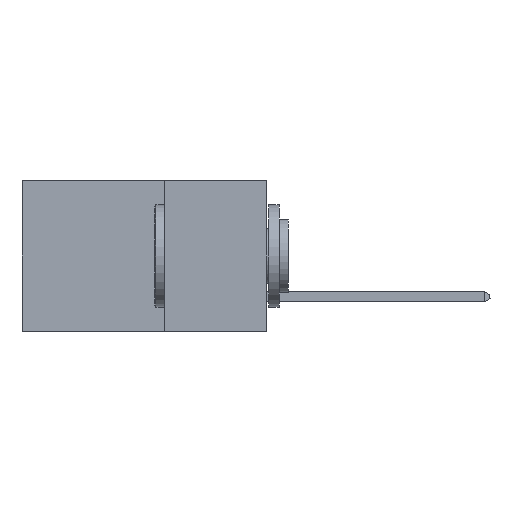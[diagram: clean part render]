
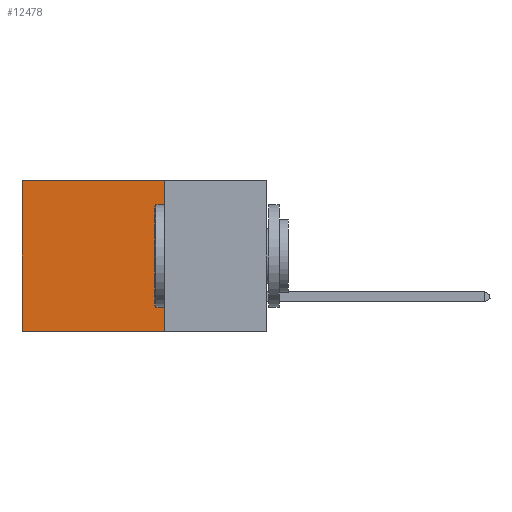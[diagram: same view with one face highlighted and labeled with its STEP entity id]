
A CAD part, left-side view. The second image highlights one B-rep face of the part: STEP entity #12478.
In plain terms, the highlighted planar face has unit normal (-1, 0, 0).
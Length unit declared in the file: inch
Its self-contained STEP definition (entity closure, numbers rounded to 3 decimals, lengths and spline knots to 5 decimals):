
#272 = DIRECTION ( 'NONE',  ( 0., 0., -1. ) ) ;
#1914 = PLANE ( 'NONE',  #24032 ) ;
#2000 = ORIENTED_EDGE ( 'NONE', *, *, #19717, .F. ) ;
#2892 = ORIENTED_EDGE ( 'NONE', *, *, #3190, .T. ) ;
#2979 = EDGE_CURVE ( 'NONE', #3474, #3676, #6004, .T. ) ;
#3190 = EDGE_CURVE ( 'NONE', #6959, #7015, #4786, .T. ) ;
#3474 = VERTEX_POINT ( 'NONE', #22950 ) ;
#3676 = VERTEX_POINT ( 'NONE', #20092 ) ;
#4786 = LINE ( 'NONE', #16646, #17984 ) ;
#4803 = VECTOR ( 'NONE', #5857, 39.37008 ) ;
#5398 = VECTOR ( 'NONE', #21744, 39.37008 ) ;
#5857 = DIRECTION ( 'NONE',  ( 0., 1., 0. ) ) ;
#5911 = CARTESIAN_POINT ( 'NONE',  ( 0.2875, 0.25, 0. ) ) ;
#6004 = LINE ( 'NONE', #17794, #5398 ) ;
#6959 = VERTEX_POINT ( 'NONE', #11608 ) ;
#7015 = VERTEX_POINT ( 'NONE', #21011 ) ;
#10780 = EDGE_CURVE ( 'NONE', #3474, #6959, #21262, .T. ) ;
#11608 = CARTESIAN_POINT ( 'NONE',  ( 0.2875, 0.6, 0. ) ) ;
#12478 = ADVANCED_FACE ( 'NONE', ( #21173 ), #1914, .F. ) ;
#15724 = DIRECTION ( 'NONE',  ( 0., 1., 0. ) ) ;
#16546 = VECTOR ( 'NONE', #15724, 39.37008 ) ;
#16646 = CARTESIAN_POINT ( 'NONE',  ( 0.2875, 0.6, 0. ) ) ;
#17124 = LINE ( 'NONE', #21621, #16546 ) ;
#17246 = ORIENTED_EDGE ( 'NONE', *, *, #10780, .T. ) ;
#17794 = CARTESIAN_POINT ( 'NONE',  ( 0.2875, 0.25, 0. ) ) ;
#17984 = VECTOR ( 'NONE', #22319, 39.37008 ) ;
#18734 = CARTESIAN_POINT ( 'NONE',  ( 0.2875, 0.25, 0. ) ) ;
#19096 = EDGE_LOOP ( 'NONE', ( #2892, #2000, #21598, #17246 ) ) ;
#19717 = EDGE_CURVE ( 'NONE', #3676, #7015, #17124, .T. ) ;
#20092 = CARTESIAN_POINT ( 'NONE',  ( 0.2875, 0.25, -0.37 ) ) ;
#20772 = DIRECTION ( 'NONE',  ( 1., 0., 0. ) ) ;
#21011 = CARTESIAN_POINT ( 'NONE',  ( 0.2875, 0.6, -0.37 ) ) ;
#21173 = FACE_OUTER_BOUND ( 'NONE', #19096, .T. ) ;
#21262 = LINE ( 'NONE', #18734, #4803 ) ;
#21598 = ORIENTED_EDGE ( 'NONE', *, *, #2979, .F. ) ;
#21621 = CARTESIAN_POINT ( 'NONE',  ( 0.2875, 0.25, -0.37 ) ) ;
#21744 = DIRECTION ( 'NONE',  ( 0., 0., -1. ) ) ;
#22319 = DIRECTION ( 'NONE',  ( 0., 0., -1. ) ) ;
#22950 = CARTESIAN_POINT ( 'NONE',  ( 0.2875, 0.25, 0. ) ) ;
#24032 = AXIS2_PLACEMENT_3D ( 'NONE', #5911, #20772, #272 ) ;
